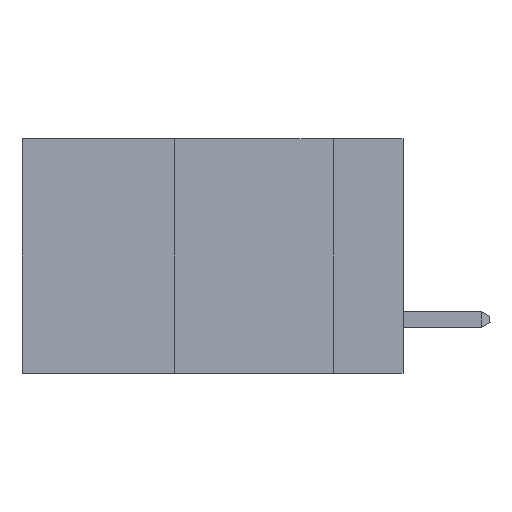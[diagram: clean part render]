
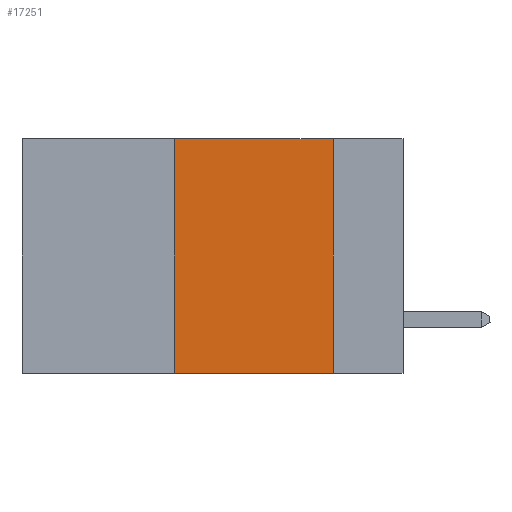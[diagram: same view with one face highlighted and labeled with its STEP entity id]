
A CAD part, left-side view. The second image highlights one B-rep face of the part: STEP entity #17251.
In plain terms, the highlighted planar face has unit normal (-1, 0, 0).
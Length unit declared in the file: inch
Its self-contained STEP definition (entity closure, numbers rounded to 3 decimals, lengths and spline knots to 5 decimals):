
#466 = VECTOR ( 'NONE', #592, 39.37008 ) ;
#592 = DIRECTION ( 'NONE',  ( 0., 0., 1. ) ) ;
#968 = VERTEX_POINT ( 'NONE', #21902 ) ;
#3143 = CARTESIAN_POINT ( 'NONE',  ( 0., 0.36, 0. ) ) ;
#3386 = DIRECTION ( 'NONE',  ( 0., 0., -1. ) ) ;
#3504 = VECTOR ( 'NONE', #16329, 39.37008 ) ;
#4136 = CARTESIAN_POINT ( 'NONE',  ( 0., 0.11, -0.37 ) ) ;
#4321 = ORIENTED_EDGE ( 'NONE', *, *, #31000, .F. ) ;
#4369 = LINE ( 'NONE', #32499, #37955 ) ;
#4567 = ORIENTED_EDGE ( 'NONE', *, *, #37256, .F. ) ;
#5494 = EDGE_CURVE ( 'NONE', #968, #15697, #23523, .T. ) ;
#6514 = AXIS2_PLACEMENT_3D ( 'NONE', #15126, #15268, #3386 ) ;
#8730 = LINE ( 'NONE', #31241, #466 ) ;
#11079 = VECTOR ( 'NONE', #13324, 39.37008 ) ;
#13254 = CARTESIAN_POINT ( 'NONE',  ( 0., 0.6, 0. ) ) ;
#13324 = DIRECTION ( 'NONE',  ( 0., -1., 0. ) ) ;
#15126 = CARTESIAN_POINT ( 'NONE',  ( 0., 0.6, 0. ) ) ;
#15268 = DIRECTION ( 'NONE',  ( 1., 0., 0. ) ) ;
#15697 = VERTEX_POINT ( 'NONE', #4136 ) ;
#16329 = DIRECTION ( 'NONE',  ( 0., -1., 0. ) ) ;
#16846 = FACE_OUTER_BOUND ( 'NONE', #29762, .T. ) ;
#17251 = ADVANCED_FACE ( 'NONE', ( #16846 ), #30126, .F. ) ;
#19493 = CARTESIAN_POINT ( 'NONE',  ( 0., 0.6, -0.37 ) ) ;
#19966 = VERTEX_POINT ( 'NONE', #3143 ) ;
#20869 = LINE ( 'NONE', #13254, #3504 ) ;
#21902 = CARTESIAN_POINT ( 'NONE',  ( 0., 0.36, -0.37 ) ) ;
#23523 = LINE ( 'NONE', #19493, #11079 ) ;
#23645 = CARTESIAN_POINT ( 'NONE',  ( 0., 0.11, 0. ) ) ;
#23725 = ORIENTED_EDGE ( 'NONE', *, *, #32230, .F. ) ;
#29762 = EDGE_LOOP ( 'NONE', ( #23725, #4321, #4567, #31964 ) ) ;
#30126 = PLANE ( 'NONE',  #6514 ) ;
#31000 = EDGE_CURVE ( 'NONE', #19966, #32968, #20869, .T. ) ;
#31241 = CARTESIAN_POINT ( 'NONE',  ( 0., 0.36, 0. ) ) ;
#31964 = ORIENTED_EDGE ( 'NONE', *, *, #5494, .T. ) ;
#32230 = EDGE_CURVE ( 'NONE', #32968, #15697, #4369, .T. ) ;
#32378 = DIRECTION ( 'NONE',  ( 0., 0., -1. ) ) ;
#32499 = CARTESIAN_POINT ( 'NONE',  ( 0., 0.11, 0. ) ) ;
#32968 = VERTEX_POINT ( 'NONE', #23645 ) ;
#37256 = EDGE_CURVE ( 'NONE', #968, #19966, #8730, .T. ) ;
#37955 = VECTOR ( 'NONE', #32378, 39.37008 ) ;
